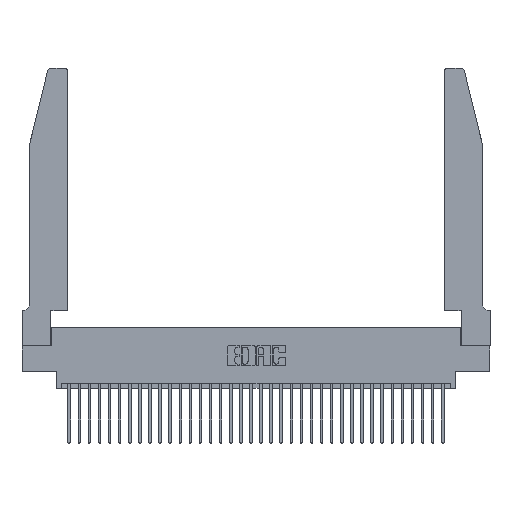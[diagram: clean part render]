
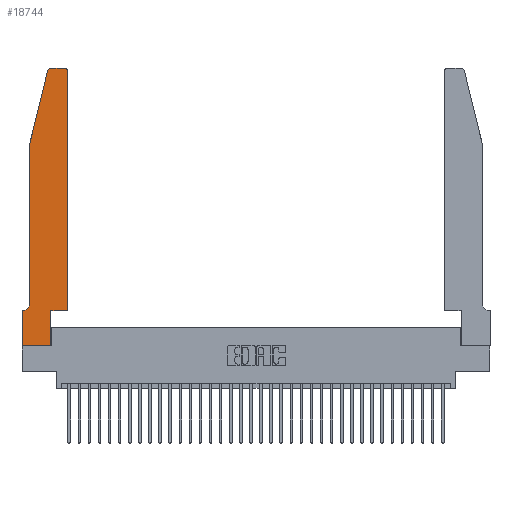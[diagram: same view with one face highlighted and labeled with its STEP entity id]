
A CAD part, top view. The second image highlights one B-rep face of the part: STEP entity #18744.
In plain terms, the highlighted planar face has unit normal (0, 0, 1).
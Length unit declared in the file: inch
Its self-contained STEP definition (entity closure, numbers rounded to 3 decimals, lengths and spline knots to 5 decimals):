
#257 = LINE ( 'NONE', #409, #21332 ) ;
#312 = EDGE_CURVE ( 'NONE', #31151, #1283, #8557, .T. ) ;
#409 = CARTESIAN_POINT ( 'NONE',  ( 0.2605, 2.75, 0.37 ) ) ;
#675 = VERTEX_POINT ( 'NONE', #26769 ) ;
#1248 = ORIENTED_EDGE ( 'NONE', *, *, #34543, .T. ) ;
#1283 = VERTEX_POINT ( 'NONE', #16351 ) ;
#1598 = LINE ( 'NONE', #16408, #16276 ) ;
#2361 = LINE ( 'NONE', #19414, #23358 ) ;
#3193 = CARTESIAN_POINT ( 'NONE',  ( 0., 0., 0.37 ) ) ;
#3199 = DIRECTION ( 'NONE',  ( -1., 0., 0. ) ) ;
#3249 = DIRECTION ( 'NONE',  ( 0., -1., 0. ) ) ;
#3376 = CARTESIAN_POINT ( 'NONE',  ( 0.0755, 0.35, 0.37 ) ) ;
#3538 = EDGE_CURVE ( 'NONE', #30038, #26004, #1598, .T. ) ;
#3615 = CARTESIAN_POINT ( 'NONE',  ( 0., 0.35, 0.37 ) ) ;
#3759 = CARTESIAN_POINT ( 'NONE',  ( 0.4505, 0.35, 0.37 ) ) ;
#3895 = CIRCLE ( 'NONE', #18155, 0.03 ) ;
#4403 = LINE ( 'NONE', #3193, #32502 ) ;
#4527 = EDGE_CURVE ( 'NONE', #26004, #675, #7180, .T. ) ;
#4728 = DIRECTION ( 'NONE',  ( 0., 0., 1. ) ) ;
#4883 = VERTEX_POINT ( 'NONE', #16928 ) ;
#5071 = CARTESIAN_POINT ( 'NONE',  ( 0.25487, 2.72718, 0.37 ) ) ;
#5135 = CARTESIAN_POINT ( 'NONE',  ( 0.0055, 0.35, 0.37 ) ) ;
#5216 = LINE ( 'NONE', #28266, #18947 ) ;
#5451 = VECTOR ( 'NONE', #6171, 39.37008 ) ;
#5622 = EDGE_CURVE ( 'NONE', #9803, #14367, #2361, .T. ) ;
#5879 = CARTESIAN_POINT ( 'NONE',  ( 0., 0., 0.37 ) ) ;
#6171 = DIRECTION ( 'NONE',  ( -1., 0., 0. ) ) ;
#6232 = CARTESIAN_POINT ( 'NONE',  ( 0.284, 2.75, 0.37 ) ) ;
#6736 = VERTEX_POINT ( 'NONE', #5071 ) ;
#7180 = LINE ( 'NONE', #7472, #27194 ) ;
#7470 = CARTESIAN_POINT ( 'NONE',  ( 0.0755, 2., 0.37 ) ) ;
#7472 = CARTESIAN_POINT ( 'NONE',  ( 0.4505, 0.35, 0.37 ) ) ;
#7913 = DIRECTION ( 'NONE',  ( 0., 0., -1. ) ) ;
#7954 = CARTESIAN_POINT ( 'NONE',  ( 0.284, 2.72, 0.37 ) ) ;
#8036 = LINE ( 'NONE', #24217, #14505 ) ;
#8557 = LINE ( 'NONE', #8949, #17593 ) ;
#8949 = CARTESIAN_POINT ( 'NONE',  ( 0.0755, 2., 0.37 ) ) ;
#9803 = VERTEX_POINT ( 'NONE', #3615 ) ;
#10685 = DIRECTION ( 'NONE',  ( 0., 1., 0. ) ) ;
#10721 = DIRECTION ( 'NONE',  ( 1., 0., 0. ) ) ;
#11414 = EDGE_CURVE ( 'NONE', #31230, #9803, #33517, .T. ) ;
#11421 = DIRECTION ( 'NONE',  ( 1., 0., 0. ) ) ;
#11790 = ORIENTED_EDGE ( 'NONE', *, *, #11414, .T. ) ;
#11936 = FACE_OUTER_BOUND ( 'NONE', #25952, .T. ) ;
#12355 = EDGE_CURVE ( 'NONE', #27197, #6736, #19607, .T. ) ;
#12455 = ORIENTED_EDGE ( 'NONE', *, *, #312, .T. ) ;
#14367 = VERTEX_POINT ( 'NONE', #5879 ) ;
#14505 = VECTOR ( 'NONE', #10685, 39.37008 ) ;
#15185 = AXIS2_PLACEMENT_3D ( 'NONE', #7954, #26986, #10721 ) ;
#15224 = ORIENTED_EDGE ( 'NONE', *, *, #3538, .T. ) ;
#16051 = CARTESIAN_POINT ( 'NONE',  ( 0.2865, 0.35, 0.37 ) ) ;
#16276 = VECTOR ( 'NONE', #35237, 39.37008 ) ;
#16351 = CARTESIAN_POINT ( 'NONE',  ( 0.0755, 0.42, 0.37 ) ) ;
#16408 = CARTESIAN_POINT ( 'NONE',  ( 0.4505, 0.35, 0.37 ) ) ;
#16928 = CARTESIAN_POINT ( 'NONE',  ( 0.4205, 2.75, 0.37 ) ) ;
#17123 = ORIENTED_EDGE ( 'NONE', *, *, #22173, .T. ) ;
#17593 = VECTOR ( 'NONE', #3249, 39.37008 ) ;
#18155 = AXIS2_PLACEMENT_3D ( 'NONE', #21144, #4728, #23840 ) ;
#18268 = CARTESIAN_POINT ( 'NONE',  ( 0.2865, 0., 0.37 ) ) ;
#18744 = ADVANCED_FACE ( 'NONE', ( #11936 ), #19412, .T. ) ;
#18947 = VECTOR ( 'NONE', #30929, 39.37008 ) ;
#19412 = PLANE ( 'NONE',  #22556 ) ;
#19414 = CARTESIAN_POINT ( 'NONE',  ( 0., 0., 0.37 ) ) ;
#19607 = CIRCLE ( 'NONE', #15185, 0.03 ) ;
#20802 = ORIENTED_EDGE ( 'NONE', *, *, #25334, .T. ) ;
#21144 = CARTESIAN_POINT ( 'NONE',  ( 0.4205, 2.72, 0.37 ) ) ;
#21332 = VECTOR ( 'NONE', #3199, 39.37008 ) ;
#22173 = EDGE_CURVE ( 'NONE', #1283, #31230, #32674, .T. ) ;
#22242 = CARTESIAN_POINT ( 'NONE',  ( 0., 0.35, 0.37 ) ) ;
#22556 = AXIS2_PLACEMENT_3D ( 'NONE', #22242, #27686, #11421 ) ;
#22752 = VERTEX_POINT ( 'NONE', #18268 ) ;
#23065 = ORIENTED_EDGE ( 'NONE', *, *, #5622, .T. ) ;
#23358 = VECTOR ( 'NONE', #24830, 39.37008 ) ;
#23840 = DIRECTION ( 'NONE',  ( 1., 0., 0. ) ) ;
#24216 = CARTESIAN_POINT ( 'NONE',  ( 0.0055, 0.42, 0.37 ) ) ;
#24217 = CARTESIAN_POINT ( 'NONE',  ( 0.2865, 0.35, 0.37 ) ) ;
#24830 = DIRECTION ( 'NONE',  ( 0., -1., 0. ) ) ;
#25334 = EDGE_CURVE ( 'NONE', #6736, #31151, #5216, .T. ) ;
#25596 = EDGE_CURVE ( 'NONE', #675, #4883, #3895, .T. ) ;
#25952 = EDGE_LOOP ( 'NONE', ( #32903, #30945, #20802, #12455, #17123, #11790, #23065, #32554, #1248, #15224, #28991, #29481 ) ) ;
#26004 = VERTEX_POINT ( 'NONE', #3759 ) ;
#26769 = CARTESIAN_POINT ( 'NONE',  ( 0.4505, 2.72, 0.37 ) ) ;
#26948 = DIRECTION ( 'NONE',  ( -1., 0., 0. ) ) ;
#26986 = DIRECTION ( 'NONE',  ( 0., 0., 1. ) ) ;
#27136 = EDGE_CURVE ( 'NONE', #14367, #22752, #4403, .T. ) ;
#27194 = VECTOR ( 'NONE', #34474, 39.37008 ) ;
#27197 = VERTEX_POINT ( 'NONE', #6232 ) ;
#27686 = DIRECTION ( 'NONE',  ( 0., 0., 1. ) ) ;
#28266 = CARTESIAN_POINT ( 'NONE',  ( 0.0755, 2., 0.37 ) ) ;
#28991 = ORIENTED_EDGE ( 'NONE', *, *, #4527, .T. ) ;
#29481 = ORIENTED_EDGE ( 'NONE', *, *, #25596, .T. ) ;
#30038 = VERTEX_POINT ( 'NONE', #16051 ) ;
#30489 = DIRECTION ( 'NONE',  ( 1., 0., 0. ) ) ;
#30895 = EDGE_CURVE ( 'NONE', #4883, #27197, #257, .T. ) ;
#30929 = DIRECTION ( 'NONE',  ( -0.239, -0.971, 0. ) ) ;
#30945 = ORIENTED_EDGE ( 'NONE', *, *, #12355, .T. ) ;
#31151 = VERTEX_POINT ( 'NONE', #7470 ) ;
#31230 = VERTEX_POINT ( 'NONE', #5135 ) ;
#32502 = VECTOR ( 'NONE', #30489, 39.37008 ) ;
#32554 = ORIENTED_EDGE ( 'NONE', *, *, #27136, .T. ) ;
#32674 = CIRCLE ( 'NONE', #34567, 0.07 ) ;
#32903 = ORIENTED_EDGE ( 'NONE', *, *, #30895, .T. ) ;
#33517 = LINE ( 'NONE', #3376, #5451 ) ;
#34474 = DIRECTION ( 'NONE',  ( 0., 1., 0. ) ) ;
#34543 = EDGE_CURVE ( 'NONE', #22752, #30038, #8036, .T. ) ;
#34567 = AXIS2_PLACEMENT_3D ( 'NONE', #24216, #7913, #26948 ) ;
#35237 = DIRECTION ( 'NONE',  ( 1., 0., 0. ) ) ;
